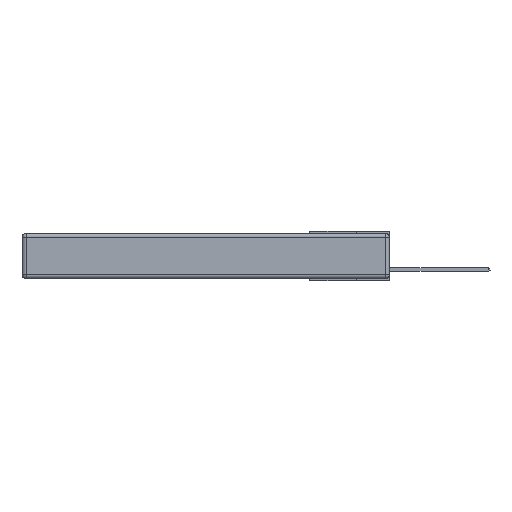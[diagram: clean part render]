
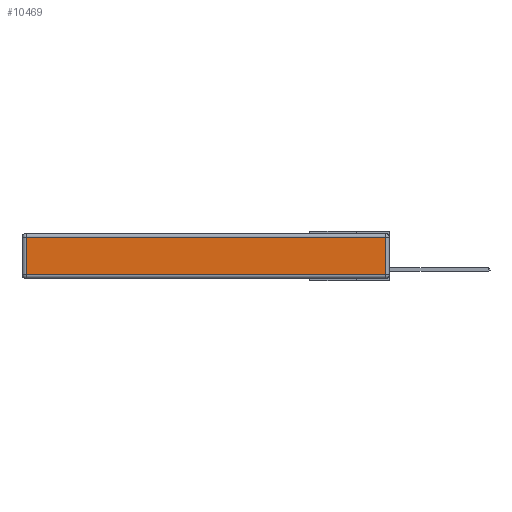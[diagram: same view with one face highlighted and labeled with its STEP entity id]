
A CAD part, left-side view. The second image highlights one B-rep face of the part: STEP entity #10469.
In plain terms, the highlighted planar face has unit normal (-1, 0, 0).
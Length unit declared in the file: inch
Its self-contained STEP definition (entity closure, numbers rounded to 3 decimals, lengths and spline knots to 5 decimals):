
#178 = PLANE ( 'NONE',  #13422 ) ;
#306 = LINE ( 'NONE', #6329, #6418 ) ;
#2387 = DIRECTION ( 'NONE',  ( 0., 1., 0. ) ) ;
#2735 = EDGE_CURVE ( 'NONE', #18132, #8905, #20230, .T. ) ;
#3493 = EDGE_CURVE ( 'NONE', #8905, #5529, #306, .T. ) ;
#4077 = LINE ( 'NONE', #7915, #21123 ) ;
#4505 = CARTESIAN_POINT ( 'NONE',  ( 0., 0.03, -0.03 ) ) ;
#4705 = ORIENTED_EDGE ( 'NONE', *, *, #2735, .T. ) ;
#5529 = VERTEX_POINT ( 'NONE', #8890 ) ;
#6048 = EDGE_LOOP ( 'NONE', ( #19136, #10600, #4705, #9707 ) ) ;
#6172 = FACE_OUTER_BOUND ( 'NONE', #6048, .T. ) ;
#6329 = CARTESIAN_POINT ( 'NONE',  ( 0., 2.72, -0.343 ) ) ;
#6418 = VECTOR ( 'NONE', #12649, 39.37008 ) ;
#7472 = CARTESIAN_POINT ( 'NONE',  ( 0., 0.03, -0.343 ) ) ;
#7915 = CARTESIAN_POINT ( 'NONE',  ( 0., 0., -0.313 ) ) ;
#7992 = LINE ( 'NONE', #7472, #14099 ) ;
#8696 = DIRECTION ( 'NONE',  ( 0., 0., 1. ) ) ;
#8890 = CARTESIAN_POINT ( 'NONE',  ( 0., 2.72, -0.313 ) ) ;
#8905 = VERTEX_POINT ( 'NONE', #15156 ) ;
#9707 = ORIENTED_EDGE ( 'NONE', *, *, #3493, .T. ) ;
#10356 = CARTESIAN_POINT ( 'NONE',  ( 0., 0., -0.343 ) ) ;
#10469 = ADVANCED_FACE ( 'NONE', ( #6172 ), #178, .T. ) ;
#10600 = ORIENTED_EDGE ( 'NONE', *, *, #16108, .T. ) ;
#11837 = CARTESIAN_POINT ( 'NONE',  ( 0., 2.75, -0.03 ) ) ;
#12649 = DIRECTION ( 'NONE',  ( 0., 0., -1. ) ) ;
#13422 = AXIS2_PLACEMENT_3D ( 'NONE', #10356, #13763, #8696 ) ;
#13763 = DIRECTION ( 'NONE',  ( -1., 0., 0. ) ) ;
#14099 = VECTOR ( 'NONE', #18868, 39.37008 ) ;
#15156 = CARTESIAN_POINT ( 'NONE',  ( 0., 2.72, -0.03 ) ) ;
#15897 = DIRECTION ( 'NONE',  ( 0., -1., 0. ) ) ;
#16058 = VERTEX_POINT ( 'NONE', #18514 ) ;
#16108 = EDGE_CURVE ( 'NONE', #16058, #18132, #7992, .T. ) ;
#16395 = VECTOR ( 'NONE', #2387, 39.37008 ) ;
#17107 = EDGE_CURVE ( 'NONE', #5529, #16058, #4077, .T. ) ;
#18132 = VERTEX_POINT ( 'NONE', #4505 ) ;
#18514 = CARTESIAN_POINT ( 'NONE',  ( 0., 0.03, -0.313 ) ) ;
#18868 = DIRECTION ( 'NONE',  ( 0., 0., 1. ) ) ;
#19136 = ORIENTED_EDGE ( 'NONE', *, *, #17107, .T. ) ;
#20230 = LINE ( 'NONE', #11837, #16395 ) ;
#21123 = VECTOR ( 'NONE', #15897, 39.37008 ) ;
